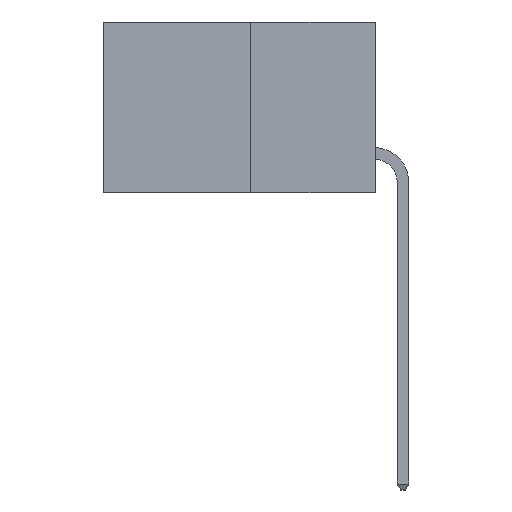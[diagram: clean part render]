
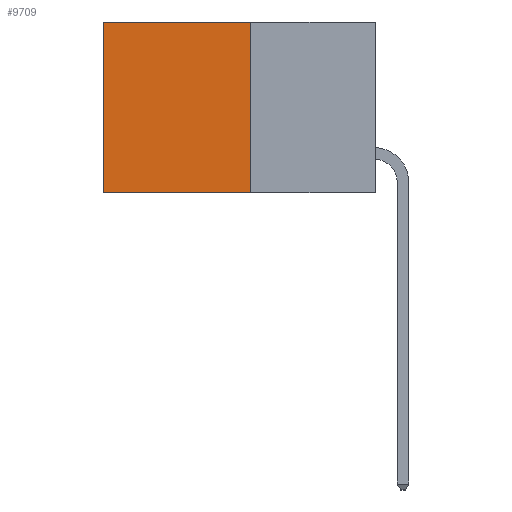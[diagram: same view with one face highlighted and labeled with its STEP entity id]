
A CAD part, left-side view. The second image highlights one B-rep face of the part: STEP entity #9709.
In plain terms, the highlighted planar face has unit normal (-1, 0, 0).
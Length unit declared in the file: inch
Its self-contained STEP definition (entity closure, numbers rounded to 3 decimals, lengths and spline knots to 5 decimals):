
#193 = DIRECTION ( 'NONE',  ( 0., 0., -1. ) ) ;
#239 = VECTOR ( 'NONE', #12920, 39.37008 ) ;
#1766 = CARTESIAN_POINT ( 'NONE',  ( 0.277, 0.27, -0.37 ) ) ;
#2884 = AXIS2_PLACEMENT_3D ( 'NONE', #6625, #12996, #193 ) ;
#3260 = EDGE_CURVE ( 'NONE', #16224, #16659, #22696, .T. ) ;
#4045 = DIRECTION ( 'NONE',  ( 0., 1., 0. ) ) ;
#4112 = CARTESIAN_POINT ( 'NONE',  ( 0.277, 0.59, 0. ) ) ;
#4982 = EDGE_CURVE ( 'NONE', #16224, #27137, #11362, .T. ) ;
#6015 = LINE ( 'NONE', #8681, #239 ) ;
#6399 = VECTOR ( 'NONE', #27565, 39.37008 ) ;
#6625 = CARTESIAN_POINT ( 'NONE',  ( 0.277, 0.27, -0.37 ) ) ;
#7358 = ORIENTED_EDGE ( 'NONE', *, *, #13185, .F. ) ;
#7686 = ORIENTED_EDGE ( 'NONE', *, *, #19111, .T. ) ;
#7805 = CARTESIAN_POINT ( 'NONE',  ( 0.277, 0.59, -0.37 ) ) ;
#7863 = CARTESIAN_POINT ( 'NONE',  ( 0.277, 0.27, 0. ) ) ;
#8681 = CARTESIAN_POINT ( 'NONE',  ( 0.277, 0.59, -0.37 ) ) ;
#8892 = LINE ( 'NONE', #1766, #25117 ) ;
#9709 = ADVANCED_FACE ( 'NONE', ( #26954 ), #10891, .F. ) ;
#10891 = PLANE ( 'NONE',  #2884 ) ;
#11362 = LINE ( 'NONE', #17439, #6399 ) ;
#12920 = DIRECTION ( 'NONE',  ( 0., 0., -1. ) ) ;
#12996 = DIRECTION ( 'NONE',  ( 1., 0., 0. ) ) ;
#13185 = EDGE_CURVE ( 'NONE', #16659, #15498, #8892, .T. ) ;
#15445 = ORIENTED_EDGE ( 'NONE', *, *, #4982, .T. ) ;
#15498 = VERTEX_POINT ( 'NONE', #7805 ) ;
#15797 = EDGE_LOOP ( 'NONE', ( #7686, #7358, #17126, #15445 ) ) ;
#16224 = VERTEX_POINT ( 'NONE', #7863 ) ;
#16659 = VERTEX_POINT ( 'NONE', #18215 ) ;
#17120 = VECTOR ( 'NONE', #25341, 39.37008 ) ;
#17126 = ORIENTED_EDGE ( 'NONE', *, *, #3260, .F. ) ;
#17439 = CARTESIAN_POINT ( 'NONE',  ( 0.277, 0.27, 0. ) ) ;
#18215 = CARTESIAN_POINT ( 'NONE',  ( 0.277, 0.27, -0.37 ) ) ;
#19111 = EDGE_CURVE ( 'NONE', #27137, #15498, #6015, .T. ) ;
#22696 = LINE ( 'NONE', #25633, #17120 ) ;
#25117 = VECTOR ( 'NONE', #4045, 39.37008 ) ;
#25341 = DIRECTION ( 'NONE',  ( 0., 0., -1. ) ) ;
#25633 = CARTESIAN_POINT ( 'NONE',  ( 0.277, 0.27, -0.37 ) ) ;
#26954 = FACE_OUTER_BOUND ( 'NONE', #15797, .T. ) ;
#27137 = VERTEX_POINT ( 'NONE', #4112 ) ;
#27565 = DIRECTION ( 'NONE',  ( 0., 1., 0. ) ) ;
